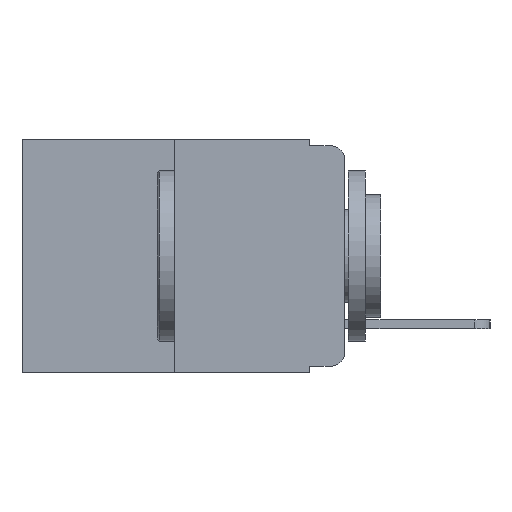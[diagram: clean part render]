
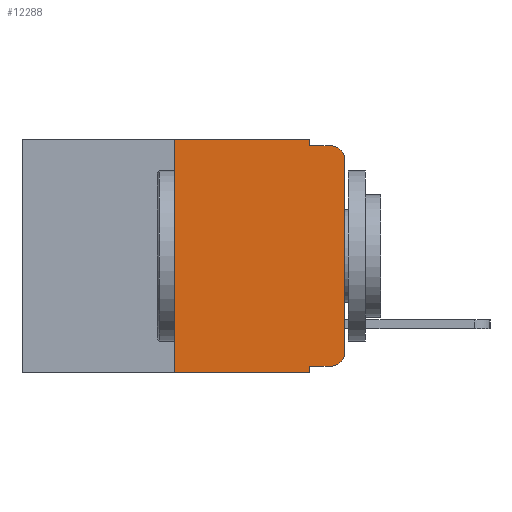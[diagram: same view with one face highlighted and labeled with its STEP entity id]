
A CAD part, left-side view. The second image highlights one B-rep face of the part: STEP entity #12288.
In plain terms, the highlighted planar face has unit normal (-1, 0, 0).
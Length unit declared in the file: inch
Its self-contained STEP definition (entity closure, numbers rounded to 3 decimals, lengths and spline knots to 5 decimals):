
#9 = EDGE_CURVE ( 'NONE', #9657, #2564, #3931, .T. ) ;
#112 = DIRECTION ( 'NONE',  ( 0., 0., -1. ) ) ;
#280 = ORIENTED_EDGE ( 'NONE', *, *, #5634, .F. ) ;
#450 = CARTESIAN_POINT ( 'NONE',  ( 0., 0.051, -0.333 ) ) ;
#766 = DIRECTION ( 'NONE',  ( 0., 0., -1. ) ) ;
#941 = FACE_OUTER_BOUND ( 'NONE', #8281, .T. ) ;
#982 = VECTOR ( 'NONE', #9701, 39.37008 ) ;
#1056 = CARTESIAN_POINT ( 'NONE',  ( 0., 0.02, -0.333 ) ) ;
#1204 = VECTOR ( 'NONE', #1905, 39.37008 ) ;
#1234 = CARTESIAN_POINT ( 'NONE',  ( 0., 0.051, 0. ) ) ;
#1360 = ORIENTED_EDGE ( 'NONE', *, *, #6903, .F. ) ;
#1413 = ORIENTED_EDGE ( 'NONE', *, *, #9, .F. ) ;
#1587 = EDGE_CURVE ( 'NONE', #6236, #1611, #2030, .T. ) ;
#1611 = VERTEX_POINT ( 'NONE', #1056 ) ;
#1905 = DIRECTION ( 'NONE',  ( 0., -1., 0. ) ) ;
#1952 = CARTESIAN_POINT ( 'NONE',  ( 0., 0.25, 0. ) ) ;
#1971 = VECTOR ( 'NONE', #12047, 39.37008 ) ;
#2030 = LINE ( 'NONE', #9999, #9119 ) ;
#2460 = AXIS2_PLACEMENT_3D ( 'NONE', #3421, #10018, #4437 ) ;
#2465 = ORIENTED_EDGE ( 'NONE', *, *, #4984, .F. ) ;
#2564 = VERTEX_POINT ( 'NONE', #5646 ) ;
#2859 = LINE ( 'NONE', #10320, #7736 ) ;
#3148 = CARTESIAN_POINT ( 'NONE',  ( 0., 0.473, 0. ) ) ;
#3280 = ORIENTED_EDGE ( 'NONE', *, *, #3996, .T. ) ;
#3421 = CARTESIAN_POINT ( 'NONE',  ( 0., 0.02, -0.03 ) ) ;
#3564 = LINE ( 'NONE', #1234, #5887 ) ;
#3595 = VERTEX_POINT ( 'NONE', #4920 ) ;
#3598 = DIRECTION ( 'NONE',  ( 0., 0., -1. ) ) ;
#3710 = LINE ( 'NONE', #1952, #982 ) ;
#3931 = LINE ( 'NONE', #3148, #1204 ) ;
#3996 = EDGE_CURVE ( 'NONE', #4714, #8143, #4683, .T. ) ;
#4158 = CARTESIAN_POINT ( 'NONE',  ( 0., 0.473, 0. ) ) ;
#4331 = EDGE_CURVE ( 'NONE', #6236, #8143, #3564, .T. ) ;
#4355 = LINE ( 'NONE', #10483, #7201 ) ;
#4437 = DIRECTION ( 'NONE',  ( 0., 0., -1. ) ) ;
#4480 = CARTESIAN_POINT ( 'NONE',  ( 0., 0., 0. ) ) ;
#4683 = LINE ( 'NONE', #7892, #1971 ) ;
#4714 = VERTEX_POINT ( 'NONE', #5038 ) ;
#4920 = CARTESIAN_POINT ( 'NONE',  ( 0., 0., -0.313 ) ) ;
#4984 = EDGE_CURVE ( 'NONE', #4714, #9657, #3710, .T. ) ;
#5038 = CARTESIAN_POINT ( 'NONE',  ( 0., 0.25, -0.343 ) ) ;
#5562 = VECTOR ( 'NONE', #6423, 39.37008 ) ;
#5634 = EDGE_CURVE ( 'NONE', #2564, #8120, #4355, .T. ) ;
#5646 = CARTESIAN_POINT ( 'NONE',  ( 0., 0.051, 0. ) ) ;
#5745 = ORIENTED_EDGE ( 'NONE', *, *, #4331, .F. ) ;
#5887 = VECTOR ( 'NONE', #3598, 39.37008 ) ;
#6009 = CIRCLE ( 'NONE', #8731, 0.02 ) ;
#6125 = DIRECTION ( 'NONE',  ( 1., 0., 0. ) ) ;
#6236 = VERTEX_POINT ( 'NONE', #450 ) ;
#6423 = DIRECTION ( 'NONE',  ( 0., 0., 1. ) ) ;
#6565 = ORIENTED_EDGE ( 'NONE', *, *, #1587, .T. ) ;
#6747 = DIRECTION ( 'NONE',  ( -1., 0., 0. ) ) ;
#6841 = ORIENTED_EDGE ( 'NONE', *, *, #10590, .T. ) ;
#6903 = EDGE_CURVE ( 'NONE', #8120, #12266, #2859, .T. ) ;
#7160 = CARTESIAN_POINT ( 'NONE',  ( 0., 0., -0.03 ) ) ;
#7201 = VECTOR ( 'NONE', #10497, 39.37008 ) ;
#7534 = CARTESIAN_POINT ( 'NONE',  ( 0., 0.051, -0.343 ) ) ;
#7691 = CARTESIAN_POINT ( 'NONE',  ( 0., 0.25, 0. ) ) ;
#7736 = VECTOR ( 'NONE', #11229, 39.37008 ) ;
#7892 = CARTESIAN_POINT ( 'NONE',  ( 0., 0.473, -0.343 ) ) ;
#8052 = LINE ( 'NONE', #4480, #5562 ) ;
#8120 = VERTEX_POINT ( 'NONE', #11167 ) ;
#8143 = VERTEX_POINT ( 'NONE', #7534 ) ;
#8281 = EDGE_LOOP ( 'NONE', ( #6841, #9712, #1360, #280, #1413, #2465, #3280, #5745, #6565, #9642 ) ) ;
#8650 = VERTEX_POINT ( 'NONE', #7160 ) ;
#8731 = AXIS2_PLACEMENT_3D ( 'NONE', #12193, #6747, #766 ) ;
#8748 = EDGE_CURVE ( 'NONE', #8650, #12266, #11094, .T. ) ;
#9119 = VECTOR ( 'NONE', #11509, 39.37008 ) ;
#9642 = ORIENTED_EDGE ( 'NONE', *, *, #10816, .T. ) ;
#9657 = VERTEX_POINT ( 'NONE', #7691 ) ;
#9701 = DIRECTION ( 'NONE',  ( 0., 0., 1. ) ) ;
#9712 = ORIENTED_EDGE ( 'NONE', *, *, #8748, .T. ) ;
#9795 = AXIS2_PLACEMENT_3D ( 'NONE', #4158, #6125, #112 ) ;
#9999 = CARTESIAN_POINT ( 'NONE',  ( 0., 0.051, -0.333 ) ) ;
#10018 = DIRECTION ( 'NONE',  ( -1., 0., 0. ) ) ;
#10320 = CARTESIAN_POINT ( 'NONE',  ( 0., 0.051, -0.01 ) ) ;
#10483 = CARTESIAN_POINT ( 'NONE',  ( 0., 0.051, 0. ) ) ;
#10497 = DIRECTION ( 'NONE',  ( 0., 0., -1. ) ) ;
#10590 = EDGE_CURVE ( 'NONE', #3595, #8650, #8052, .T. ) ;
#10816 = EDGE_CURVE ( 'NONE', #1611, #3595, #6009, .T. ) ;
#11094 = CIRCLE ( 'NONE', #2460, 0.02 ) ;
#11167 = CARTESIAN_POINT ( 'NONE',  ( 0., 0.051, -0.01 ) ) ;
#11229 = DIRECTION ( 'NONE',  ( 0., -1., 0. ) ) ;
#11509 = DIRECTION ( 'NONE',  ( 0., -1., 0. ) ) ;
#11562 = CARTESIAN_POINT ( 'NONE',  ( 0., 0.02, -0.01 ) ) ;
#11599 = PLANE ( 'NONE',  #9795 ) ;
#12047 = DIRECTION ( 'NONE',  ( 0., -1., 0. ) ) ;
#12193 = CARTESIAN_POINT ( 'NONE',  ( 0., 0.02, -0.313 ) ) ;
#12266 = VERTEX_POINT ( 'NONE', #11562 ) ;
#12288 = ADVANCED_FACE ( 'NONE', ( #941 ), #11599, .F. ) ;
